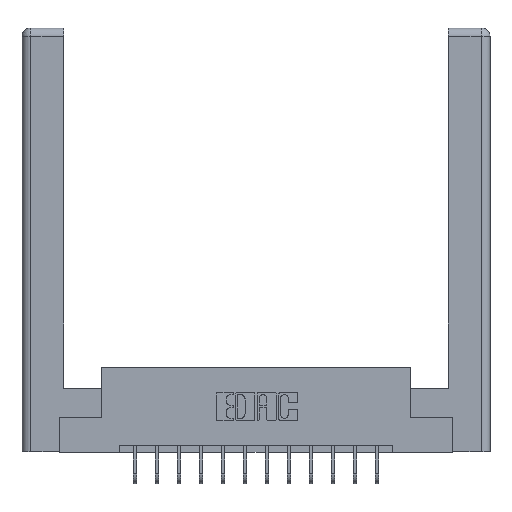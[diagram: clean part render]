
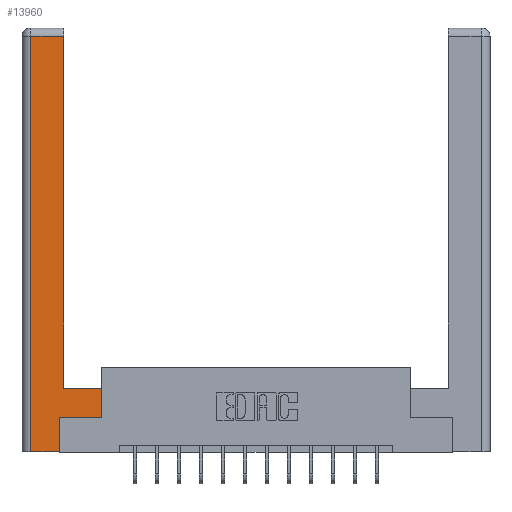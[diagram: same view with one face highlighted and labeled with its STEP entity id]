
A CAD part, top view. The second image highlights one B-rep face of the part: STEP entity #13960.
In plain terms, the highlighted planar face has unit normal (0, 0, 1).
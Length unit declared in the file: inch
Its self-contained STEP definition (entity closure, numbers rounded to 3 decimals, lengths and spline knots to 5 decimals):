
#319 = CARTESIAN_POINT ( 'NONE',  ( 0.565, 0.45, 0. ) ) ;
#653 = CARTESIAN_POINT ( 'NONE',  ( 0.565, 0.245, 0. ) ) ;
#1774 = EDGE_CURVE ( 'NONE', #8581, #10904, #13142, .T. ) ;
#1834 = ORIENTED_EDGE ( 'NONE', *, *, #13662, .T. ) ;
#1962 = CARTESIAN_POINT ( 'NONE',  ( 0., 0., 0. ) ) ;
#2232 = CARTESIAN_POINT ( 'NONE',  ( 0.565, 0.245, 0. ) ) ;
#2356 = VERTEX_POINT ( 'NONE', #3591 ) ;
#2385 = VECTOR ( 'NONE', #16895, 39.37008 ) ;
#2692 = VERTEX_POINT ( 'NONE', #3250 ) ;
#2756 = DIRECTION ( 'NONE',  ( 0., 1., 0. ) ) ;
#2831 = DIRECTION ( 'NONE',  ( -1., 0., 0. ) ) ;
#3250 = CARTESIAN_POINT ( 'NONE',  ( 0.265, 0., 0. ) ) ;
#3460 = CARTESIAN_POINT ( 'NONE',  ( 0.295, 0.45, 0. ) ) ;
#3591 = CARTESIAN_POINT ( 'NONE',  ( 0.0615, 2.94, 0. ) ) ;
#3900 = CARTESIAN_POINT ( 'NONE',  ( 0.295, 2.94, 0. ) ) ;
#4332 = FACE_OUTER_BOUND ( 'NONE', #17139, .T. ) ;
#4829 = EDGE_CURVE ( 'NONE', #13128, #8581, #16892, .T. ) ;
#4984 = ORIENTED_EDGE ( 'NONE', *, *, #16065, .T. ) ;
#5174 = CARTESIAN_POINT ( 'NONE',  ( 0.0615, 0., 0. ) ) ;
#5571 = CARTESIAN_POINT ( 'NONE',  ( 0.295, 0.45, 0. ) ) ;
#5805 = CARTESIAN_POINT ( 'NONE',  ( 0.265, 0.245, 0. ) ) ;
#5895 = CARTESIAN_POINT ( 'NONE',  ( 0.265, 0., 0. ) ) ;
#6069 = CARTESIAN_POINT ( 'NONE',  ( 0.265, 0.245, 0. ) ) ;
#6085 = DIRECTION ( 'NONE',  ( 1., 0., 0. ) ) ;
#6712 = ORIENTED_EDGE ( 'NONE', *, *, #15055, .T. ) ;
#6761 = VERTEX_POINT ( 'NONE', #12300 ) ;
#6933 = LINE ( 'NONE', #5805, #13264 ) ;
#7005 = DIRECTION ( 'NONE',  ( 1., 0., 0. ) ) ;
#7019 = CARTESIAN_POINT ( 'NONE',  ( 0.565, 0.45, 0. ) ) ;
#7488 = DIRECTION ( 'NONE',  ( 0., 0., -1. ) ) ;
#7516 = LINE ( 'NONE', #7019, #10264 ) ;
#8375 = EDGE_CURVE ( 'NONE', #10904, #2356, #15364, .T. ) ;
#8581 = VERTEX_POINT ( 'NONE', #3460 ) ;
#8921 = VECTOR ( 'NONE', #6085, 39.37008 ) ;
#9035 = VERTEX_POINT ( 'NONE', #6069 ) ;
#9611 = DIRECTION ( 'NONE',  ( 0., 1., 0. ) ) ;
#10264 = VECTOR ( 'NONE', #2756, 39.37008 ) ;
#10559 = DIRECTION ( 'NONE',  ( 0., -1., 0. ) ) ;
#10648 = LINE ( 'NONE', #5895, #13180 ) ;
#10904 = VERTEX_POINT ( 'NONE', #3900 ) ;
#12300 = CARTESIAN_POINT ( 'NONE',  ( 0.0615, 0., 0. ) ) ;
#12316 = EDGE_CURVE ( 'NONE', #2692, #9035, #6933, .T. ) ;
#12485 = ORIENTED_EDGE ( 'NONE', *, *, #4829, .T. ) ;
#12854 = DIRECTION ( 'NONE',  ( -1., 0., 0. ) ) ;
#13128 = VERTEX_POINT ( 'NONE', #319 ) ;
#13142 = LINE ( 'NONE', #16825, #15941 ) ;
#13180 = VECTOR ( 'NONE', #7005, 39.37008 ) ;
#13264 = VECTOR ( 'NONE', #16840, 39.37008 ) ;
#13662 = EDGE_CURVE ( 'NONE', #16602, #13128, #7516, .T. ) ;
#13960 = ADVANCED_FACE ( 'NONE', ( #4332 ), #17117, .F. ) ;
#14156 = CARTESIAN_POINT ( 'NONE',  ( 0.0615, 2.94, 0. ) ) ;
#14342 = VECTOR ( 'NONE', #2831, 39.37008 ) ;
#14686 = LINE ( 'NONE', #5174, #15130 ) ;
#14779 = EDGE_CURVE ( 'NONE', #2356, #6761, #14686, .T. ) ;
#15044 = ORIENTED_EDGE ( 'NONE', *, *, #1774, .T. ) ;
#15055 = EDGE_CURVE ( 'NONE', #6761, #2692, #10648, .T. ) ;
#15130 = VECTOR ( 'NONE', #10559, 39.37008 ) ;
#15285 = ORIENTED_EDGE ( 'NONE', *, *, #8375, .T. ) ;
#15291 = ORIENTED_EDGE ( 'NONE', *, *, #14779, .T. ) ;
#15364 = LINE ( 'NONE', #14156, #2385 ) ;
#15562 = ORIENTED_EDGE ( 'NONE', *, *, #12316, .T. ) ;
#15941 = VECTOR ( 'NONE', #9611, 39.37008 ) ;
#16065 = EDGE_CURVE ( 'NONE', #9035, #16602, #17023, .T. ) ;
#16602 = VERTEX_POINT ( 'NONE', #2232 ) ;
#16825 = CARTESIAN_POINT ( 'NONE',  ( 0.295, 3., 0. ) ) ;
#16840 = DIRECTION ( 'NONE',  ( 0., 1., 0. ) ) ;
#16892 = LINE ( 'NONE', #5571, #14342 ) ;
#16895 = DIRECTION ( 'NONE',  ( -1., 0., 0. ) ) ;
#17013 = AXIS2_PLACEMENT_3D ( 'NONE', #1962, #7488, #12854 ) ;
#17023 = LINE ( 'NONE', #653, #8921 ) ;
#17117 = PLANE ( 'NONE',  #17013 ) ;
#17139 = EDGE_LOOP ( 'NONE', ( #15044, #15285, #15291, #6712, #15562, #4984, #1834, #12485 ) ) ;
